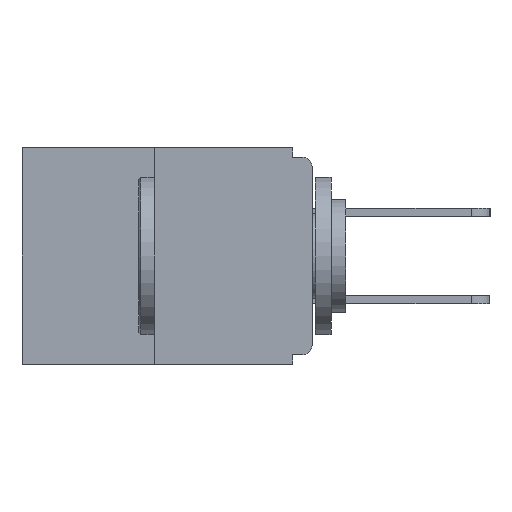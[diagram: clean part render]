
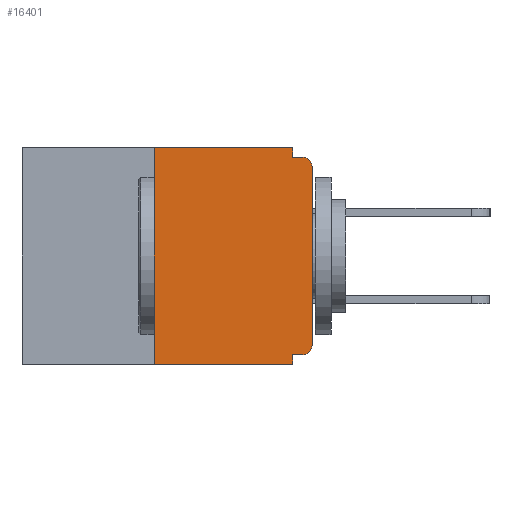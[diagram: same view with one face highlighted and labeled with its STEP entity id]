
A CAD part, left-side view. The second image highlights one B-rep face of the part: STEP entity #16401.
In plain terms, the highlighted planar face has unit normal (-1, 0, 0).
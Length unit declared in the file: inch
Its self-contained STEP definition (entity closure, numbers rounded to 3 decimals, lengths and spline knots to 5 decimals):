
#355 = CARTESIAN_POINT ( 'NONE',  ( 0., 0.031, 0. ) ) ;
#704 = CARTESIAN_POINT ( 'NONE',  ( 0., 0.25, 0. ) ) ;
#1019 = EDGE_CURVE ( 'NONE', #11420, #5847, #14961, .T. ) ;
#1325 = VERTEX_POINT ( 'NONE', #5734 ) ;
#1623 = EDGE_CURVE ( 'NONE', #4590, #2315, #1744, .T. ) ;
#1684 = LINE ( 'NONE', #14786, #7555 ) ;
#1744 = LINE ( 'NONE', #6727, #12899 ) ;
#1890 = EDGE_CURVE ( 'NONE', #12590, #2315, #12884, .T. ) ;
#2272 = EDGE_CURVE ( 'NONE', #16037, #2398, #8016, .T. ) ;
#2315 = VERTEX_POINT ( 'NONE', #12802 ) ;
#2398 = VERTEX_POINT ( 'NONE', #355 ) ;
#2621 = LINE ( 'NONE', #12672, #5627 ) ;
#3170 = EDGE_CURVE ( 'NONE', #12590, #16037, #11382, .T. ) ;
#3253 = EDGE_CURVE ( 'NONE', #2398, #16554, #9543, .T. ) ;
#3454 = CARTESIAN_POINT ( 'NONE',  ( 0., 0., -0.313 ) ) ;
#3688 = VECTOR ( 'NONE', #9711, 39.37008 ) ;
#4014 = EDGE_CURVE ( 'NONE', #4725, #4590, #2621, .T. ) ;
#4563 = ORIENTED_EDGE ( 'NONE', *, *, #15882, .T. ) ;
#4590 = VERTEX_POINT ( 'NONE', #13097 ) ;
#4725 = VERTEX_POINT ( 'NONE', #4861 ) ;
#4734 = CIRCLE ( 'NONE', #9770, 0.015 ) ;
#4861 = CARTESIAN_POINT ( 'NONE',  ( 0., 0.015, -0.328 ) ) ;
#4920 = CARTESIAN_POINT ( 'NONE',  ( 0., 0.015, -0.313 ) ) ;
#4965 = DIRECTION ( 'NONE',  ( 0., 0., -1. ) ) ;
#5415 = ORIENTED_EDGE ( 'NONE', *, *, #3170, .F. ) ;
#5497 = ORIENTED_EDGE ( 'NONE', *, *, #7448, .T. ) ;
#5627 = VECTOR ( 'NONE', #12923, 39.37008 ) ;
#5687 = VECTOR ( 'NONE', #9220, 39.37008 ) ;
#5734 = CARTESIAN_POINT ( 'NONE',  ( 0., 0.015, -0.015 ) ) ;
#5847 = VERTEX_POINT ( 'NONE', #12527 ) ;
#6307 = DIRECTION ( 'NONE',  ( 0., 0., 1. ) ) ;
#6727 = CARTESIAN_POINT ( 'NONE',  ( 0., 0.031, -0.343 ) ) ;
#6846 = DIRECTION ( 'NONE',  ( 0., 0., -1. ) ) ;
#6998 = DIRECTION ( 'NONE',  ( -1., 0., 0. ) ) ;
#7026 = DIRECTION ( 'NONE',  ( 0., 0., -1. ) ) ;
#7448 = EDGE_CURVE ( 'NONE', #4725, #11420, #12684, .T. ) ;
#7455 = CARTESIAN_POINT ( 'NONE',  ( 0., 0.46, 0. ) ) ;
#7555 = VECTOR ( 'NONE', #10927, 39.37008 ) ;
#7588 = VECTOR ( 'NONE', #8724, 39.37008 ) ;
#7778 = EDGE_LOOP ( 'NONE', ( #11033, #5415, #9809, #8284, #16676, #5497, #12376, #4563, #14418, #12848 ) ) ;
#8016 = LINE ( 'NONE', #16692, #9055 ) ;
#8109 = AXIS2_PLACEMENT_3D ( 'NONE', #4920, #12621, #7026 ) ;
#8284 = ORIENTED_EDGE ( 'NONE', *, *, #1623, .F. ) ;
#8663 = CARTESIAN_POINT ( 'NONE',  ( 0., 0.46, -0.343 ) ) ;
#8724 = DIRECTION ( 'NONE',  ( 0., -1., 0. ) ) ;
#9055 = VECTOR ( 'NONE', #12860, 39.37008 ) ;
#9220 = DIRECTION ( 'NONE',  ( 0., 0., -1. ) ) ;
#9543 = LINE ( 'NONE', #15936, #5687 ) ;
#9711 = DIRECTION ( 'NONE',  ( 0., 0., 1. ) ) ;
#9736 = CARTESIAN_POINT ( 'NONE',  ( 0., 0.015, -0.03 ) ) ;
#9770 = AXIS2_PLACEMENT_3D ( 'NONE', #9736, #6998, #16113 ) ;
#9809 = ORIENTED_EDGE ( 'NONE', *, *, #1890, .T. ) ;
#10447 = CARTESIAN_POINT ( 'NONE',  ( 0., 0.25, -0.343 ) ) ;
#10872 = CARTESIAN_POINT ( 'NONE',  ( 0., 0.031, -0.015 ) ) ;
#10927 = DIRECTION ( 'NONE',  ( 0., -1., 0. ) ) ;
#11033 = ORIENTED_EDGE ( 'NONE', *, *, #2272, .F. ) ;
#11382 = LINE ( 'NONE', #704, #3688 ) ;
#11420 = VERTEX_POINT ( 'NONE', #3454 ) ;
#11501 = CARTESIAN_POINT ( 'NONE',  ( 0., 0., 0. ) ) ;
#12239 = CARTESIAN_POINT ( 'NONE',  ( 0., 0.25, 0. ) ) ;
#12376 = ORIENTED_EDGE ( 'NONE', *, *, #1019, .T. ) ;
#12527 = CARTESIAN_POINT ( 'NONE',  ( 0., 0., -0.03 ) ) ;
#12590 = VERTEX_POINT ( 'NONE', #10447 ) ;
#12605 = PLANE ( 'NONE',  #16448 ) ;
#12621 = DIRECTION ( 'NONE',  ( -1., 0., 0. ) ) ;
#12672 = CARTESIAN_POINT ( 'NONE',  ( 0., 0., -0.328 ) ) ;
#12684 = CIRCLE ( 'NONE', #8109, 0.015 ) ;
#12802 = CARTESIAN_POINT ( 'NONE',  ( 0., 0.031, -0.343 ) ) ;
#12848 = ORIENTED_EDGE ( 'NONE', *, *, #3253, .F. ) ;
#12860 = DIRECTION ( 'NONE',  ( 0., -1., 0. ) ) ;
#12884 = LINE ( 'NONE', #8663, #7588 ) ;
#12899 = VECTOR ( 'NONE', #6846, 39.37008 ) ;
#12923 = DIRECTION ( 'NONE',  ( 0., 1., 0. ) ) ;
#13097 = CARTESIAN_POINT ( 'NONE',  ( 0., 0.031, -0.328 ) ) ;
#14107 = DIRECTION ( 'NONE',  ( 1., 0., 0. ) ) ;
#14351 = VECTOR ( 'NONE', #6307, 39.37008 ) ;
#14418 = ORIENTED_EDGE ( 'NONE', *, *, #15758, .F. ) ;
#14786 = CARTESIAN_POINT ( 'NONE',  ( 0., 0., -0.015 ) ) ;
#14961 = LINE ( 'NONE', #11501, #14351 ) ;
#15758 = EDGE_CURVE ( 'NONE', #16554, #1325, #1684, .T. ) ;
#15882 = EDGE_CURVE ( 'NONE', #5847, #1325, #4734, .T. ) ;
#15886 = FACE_OUTER_BOUND ( 'NONE', #7778, .T. ) ;
#15936 = CARTESIAN_POINT ( 'NONE',  ( 0., 0.031, 0. ) ) ;
#16037 = VERTEX_POINT ( 'NONE', #12239 ) ;
#16113 = DIRECTION ( 'NONE',  ( 0., 0., -1. ) ) ;
#16401 = ADVANCED_FACE ( 'NONE', ( #15886 ), #12605, .F. ) ;
#16448 = AXIS2_PLACEMENT_3D ( 'NONE', #7455, #14107, #4965 ) ;
#16554 = VERTEX_POINT ( 'NONE', #10872 ) ;
#16676 = ORIENTED_EDGE ( 'NONE', *, *, #4014, .F. ) ;
#16692 = CARTESIAN_POINT ( 'NONE',  ( 0., 0.46, 0. ) ) ;
